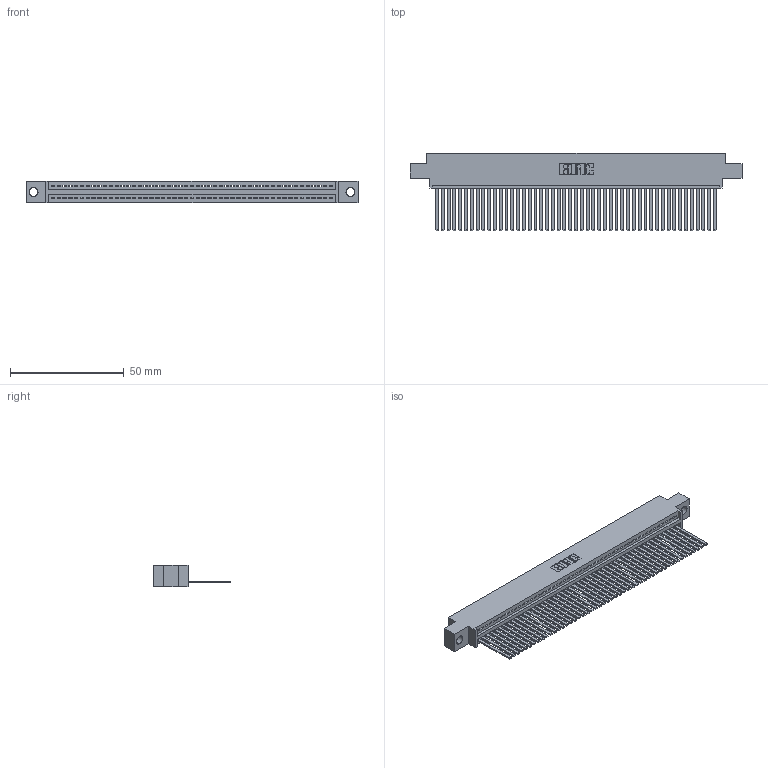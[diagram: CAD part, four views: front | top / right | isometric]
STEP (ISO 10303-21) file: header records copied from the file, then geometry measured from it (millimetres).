
FILE_DESCRIPTION (( 'STEP AP203' ), '1' );
FILE_NAME ('395-049-544-604.STEP', '2021-05-31T15:20:16', ( '' ), ( '' ), 'SwSTEP 2.0', 'SolidWorks 2020', '' );
FILE_SCHEMA (( 'CONFIG_CONTROL_DESIGN' ));
Length unit declared in the file: inch
Products named in the file (3): 395-049-544-604; 345 Part_0.170 Offset - 0.156 Dia-TI; 345-292-001_345-293-144
Assembly tree (50 placements, depth 2):
  395-049-544-604
    345 Part_0.170 Offset - 0.156 Dia-TI
    345-292-001_345-293-144  x49
Bounding box: 145.67 x 33.96 x 9.4 mm (x, y, z)
Volume: 14241.3 mm3; surface area: 20693.2 mm2
Topology: 50 solids, 50 shells, 2692 faces, 8131 edges, 5354 vertices
Faces by surface type: plane 1862, cylinder 830
Entity records: 36303 total; most frequent: CARTESIAN_POINT 6297, ORIENTED_EDGE 6278, DIRECTION 5485, EDGE_CURVE 3139, LINE 2815, VECTOR 2815, VERTEX_POINT 2090, AXIS2_PLACEMENT_3D 1335
